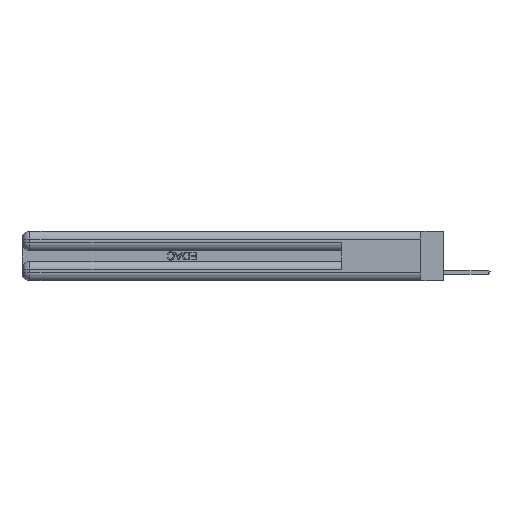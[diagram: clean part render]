
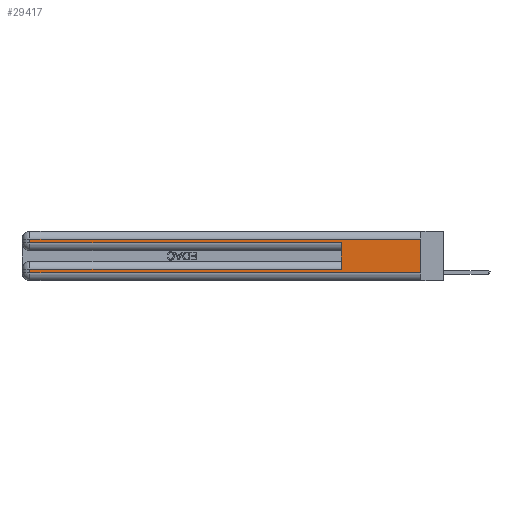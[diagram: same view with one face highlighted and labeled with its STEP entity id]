
A CAD part, left-side view. The second image highlights one B-rep face of the part: STEP entity #29417.
In plain terms, the highlighted planar face has unit normal (-1, 0, 0).
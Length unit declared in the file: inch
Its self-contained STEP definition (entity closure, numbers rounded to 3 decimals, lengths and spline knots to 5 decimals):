
#844 = VECTOR ( 'NONE', #30625, 39.37008 ) ;
#1175 = VERTEX_POINT ( 'NONE', #16880 ) ;
#2660 = CARTESIAN_POINT ( 'NONE',  ( 0., 0., 0.085 ) ) ;
#4289 = CARTESIAN_POINT ( 'NONE',  ( 0., 0., 0.31 ) ) ;
#4359 = CARTESIAN_POINT ( 'NONE',  ( 0., 0., 0.285 ) ) ;
#4444 = EDGE_LOOP ( 'NONE', ( #25143, #24703, #31251, #22633, #6914, #31446, #32767, #30990 ) ) ;
#4935 = VECTOR ( 'NONE', #18792, 39.37008 ) ;
#5454 = CARTESIAN_POINT ( 'NONE',  ( 0., 0.6, 0.085 ) ) ;
#5784 = DIRECTION ( 'NONE',  ( 0., 0., -1. ) ) ;
#6914 = ORIENTED_EDGE ( 'NONE', *, *, #14042, .F. ) ;
#6978 = DIRECTION ( 'NONE',  ( 0., -1., 0. ) ) ;
#7918 = DIRECTION ( 'NONE',  ( 0., 0., -1. ) ) ;
#9060 = EDGE_CURVE ( 'NONE', #22607, #1175, #21410, .T. ) ;
#9373 = CARTESIAN_POINT ( 'NONE',  ( 0., 0., 0.06 ) ) ;
#10576 = VECTOR ( 'NONE', #5784, 39.37008 ) ;
#10952 = CARTESIAN_POINT ( 'NONE',  ( 0., 2.94, 0.37 ) ) ;
#11123 = LINE ( 'NONE', #26568, #4935 ) ;
#11991 = VERTEX_POINT ( 'NONE', #28481 ) ;
#12584 = EDGE_CURVE ( 'NONE', #14845, #11991, #17434, .T. ) ;
#12751 = PLANE ( 'NONE',  #14264 ) ;
#13440 = CARTESIAN_POINT ( 'NONE',  ( 0., 2.94, 0.31 ) ) ;
#13635 = DIRECTION ( 'NONE',  ( 0., 0., -1. ) ) ;
#13917 = CARTESIAN_POINT ( 'NONE',  ( 0., 0., 0.31 ) ) ;
#14022 = VECTOR ( 'NONE', #13635, 39.37008 ) ;
#14042 = EDGE_CURVE ( 'NONE', #32740, #23606, #11123, .T. ) ;
#14264 = AXIS2_PLACEMENT_3D ( 'NONE', #31308, #26068, #21084 ) ;
#14845 = VERTEX_POINT ( 'NONE', #33151 ) ;
#14862 = LINE ( 'NONE', #4359, #33123 ) ;
#16094 = LINE ( 'NONE', #13917, #29406 ) ;
#16696 = EDGE_CURVE ( 'NONE', #22421, #14845, #21480, .T. ) ;
#16880 = CARTESIAN_POINT ( 'NONE',  ( 0., 2.94, 0.285 ) ) ;
#17434 = LINE ( 'NONE', #9373, #844 ) ;
#18792 = DIRECTION ( 'NONE',  ( 0., 0., 1. ) ) ;
#20384 = DIRECTION ( 'NONE',  ( 0., 1., 0. ) ) ;
#21084 = DIRECTION ( 'NONE',  ( 0., 0., -1. ) ) ;
#21207 = DIRECTION ( 'NONE',  ( 0., 1., 0. ) ) ;
#21410 = LINE ( 'NONE', #29156, #33433 ) ;
#21480 = LINE ( 'NONE', #10952, #14022 ) ;
#22421 = VERTEX_POINT ( 'NONE', #28418 ) ;
#22607 = VERTEX_POINT ( 'NONE', #13440 ) ;
#22633 = ORIENTED_EDGE ( 'NONE', *, *, #30515, .T. ) ;
#23606 = VERTEX_POINT ( 'NONE', #29231 ) ;
#24703 = ORIENTED_EDGE ( 'NONE', *, *, #25576, .T. ) ;
#25143 = ORIENTED_EDGE ( 'NONE', *, *, #32217, .F. ) ;
#25576 = EDGE_CURVE ( 'NONE', #31688, #22607, #16094, .T. ) ;
#26068 = DIRECTION ( 'NONE',  ( 1., 0., 0. ) ) ;
#26313 = LINE ( 'NONE', #2660, #33763 ) ;
#26568 = CARTESIAN_POINT ( 'NONE',  ( 0., 0.6, 0.145 ) ) ;
#28028 = CARTESIAN_POINT ( 'NONE',  ( 0., 0., 0.37 ) ) ;
#28418 = CARTESIAN_POINT ( 'NONE',  ( 0., 2.94, 0.085 ) ) ;
#28481 = CARTESIAN_POINT ( 'NONE',  ( 0., 0., 0.06 ) ) ;
#29156 = CARTESIAN_POINT ( 'NONE',  ( 0., 2.94, 0.37 ) ) ;
#29231 = CARTESIAN_POINT ( 'NONE',  ( 0., 0.6, 0.285 ) ) ;
#29406 = VECTOR ( 'NONE', #20384, 39.37008 ) ;
#29417 = ADVANCED_FACE ( 'NONE', ( #34064 ), #12751, .F. ) ;
#30515 = EDGE_CURVE ( 'NONE', #1175, #23606, #14862, .T. ) ;
#30625 = DIRECTION ( 'NONE',  ( 0., -1., 0. ) ) ;
#30990 = ORIENTED_EDGE ( 'NONE', *, *, #12584, .T. ) ;
#31251 = ORIENTED_EDGE ( 'NONE', *, *, #9060, .T. ) ;
#31308 = CARTESIAN_POINT ( 'NONE',  ( 0., 0., 0.37 ) ) ;
#31446 = ORIENTED_EDGE ( 'NONE', *, *, #32662, .T. ) ;
#31688 = VERTEX_POINT ( 'NONE', #4289 ) ;
#32217 = EDGE_CURVE ( 'NONE', #31688, #11991, #33795, .T. ) ;
#32662 = EDGE_CURVE ( 'NONE', #32740, #22421, #26313, .T. ) ;
#32740 = VERTEX_POINT ( 'NONE', #5454 ) ;
#32767 = ORIENTED_EDGE ( 'NONE', *, *, #16696, .T. ) ;
#33123 = VECTOR ( 'NONE', #6978, 39.37008 ) ;
#33151 = CARTESIAN_POINT ( 'NONE',  ( 0., 2.94, 0.06 ) ) ;
#33433 = VECTOR ( 'NONE', #7918, 39.37008 ) ;
#33763 = VECTOR ( 'NONE', #21207, 39.37008 ) ;
#33795 = LINE ( 'NONE', #28028, #10576 ) ;
#34064 = FACE_OUTER_BOUND ( 'NONE', #4444, .T. ) ;
